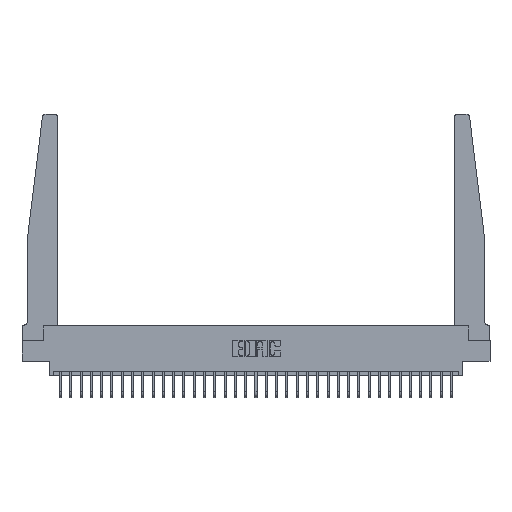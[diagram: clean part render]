
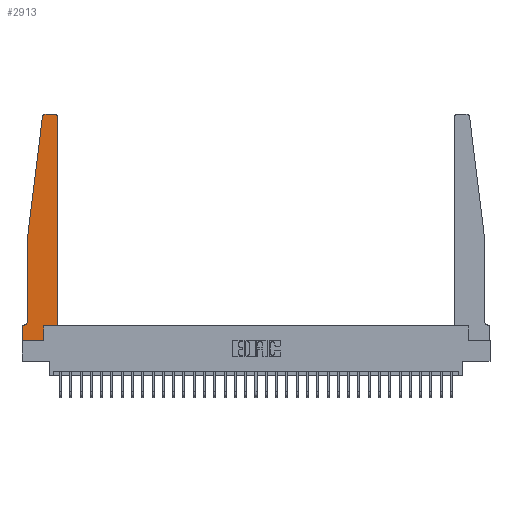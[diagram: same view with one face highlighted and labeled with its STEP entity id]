
A CAD part, top view. The second image highlights one B-rep face of the part: STEP entity #2913.
In plain terms, the highlighted planar face has unit normal (0, 0, 1).
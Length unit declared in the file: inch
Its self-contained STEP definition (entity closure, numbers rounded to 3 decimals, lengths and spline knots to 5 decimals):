
#86 = VERTEX_POINT ( 'NONE', #5348 ) ;
#124 = EDGE_CURVE ( 'NONE', #28373, #17568, #4726, .T. ) ;
#569 = CARTESIAN_POINT ( 'NONE',  ( 0.425, 0.18, 0.37 ) ) ;
#706 = VECTOR ( 'NONE', #23065, 39.37008 ) ;
#1404 = DIRECTION ( 'NONE',  ( -0.122, -0.992, 0. ) ) ;
#1860 = VERTEX_POINT ( 'NONE', #11119 ) ;
#1954 = LINE ( 'NONE', #28552, #3933 ) ;
#2847 = CARTESIAN_POINT ( 'NONE',  ( 0.015, 0.1875, 0.37 ) ) ;
#2901 = EDGE_CURVE ( 'NONE', #11012, #7720, #5055, .T. ) ;
#2913 = ADVANCED_FACE ( 'NONE', ( #12912 ), #19664, .T. ) ;
#3160 = CARTESIAN_POINT ( 'NONE',  ( 0., 0., 0.37 ) ) ;
#3933 = VECTOR ( 'NONE', #21158, 39.37008 ) ;
#4501 = CARTESIAN_POINT ( 'NONE',  ( 0.25, 2.75, 0.37 ) ) ;
#4514 = DIRECTION ( 'NONE',  ( 0., 0., 1. ) ) ;
#4726 = LINE ( 'NONE', #18181, #706 ) ;
#5055 = CIRCLE ( 'NONE', #15534, 0.03 ) ;
#5106 = EDGE_CURVE ( 'NONE', #86, #31598, #19056, .T. ) ;
#5206 = EDGE_CURVE ( 'NONE', #7720, #86, #7286, .T. ) ;
#5348 = CARTESIAN_POINT ( 'NONE',  ( 0.065, 1.25, 0.37 ) ) ;
#5720 = VECTOR ( 'NONE', #13809, 39.37008 ) ;
#5802 = ORIENTED_EDGE ( 'NONE', *, *, #2901, .T. ) ;
#5968 = LINE ( 'NONE', #26491, #18101 ) ;
#6328 = DIRECTION ( 'NONE',  ( 0., -1., 0. ) ) ;
#6398 = ORIENTED_EDGE ( 'NONE', *, *, #15980, .T. ) ;
#7286 = LINE ( 'NONE', #26779, #8465 ) ;
#7720 = VERTEX_POINT ( 'NONE', #19216 ) ;
#7993 = EDGE_CURVE ( 'NONE', #17568, #1860, #5968, .T. ) ;
#8465 = VECTOR ( 'NONE', #1404, 39.37008 ) ;
#8578 = VERTEX_POINT ( 'NONE', #11806 ) ;
#9713 = CARTESIAN_POINT ( 'NONE',  ( 0.27653, 2.72, 0.37 ) ) ;
#10337 = VECTOR ( 'NONE', #14319, 39.37008 ) ;
#11012 = VERTEX_POINT ( 'NONE', #11252 ) ;
#11119 = CARTESIAN_POINT ( 'NONE',  ( 0.2605, 0.18, 0.37 ) ) ;
#11252 = CARTESIAN_POINT ( 'NONE',  ( 0.27653, 2.75, 0.37 ) ) ;
#11569 = VECTOR ( 'NONE', #6328, 39.37008 ) ;
#11806 = CARTESIAN_POINT ( 'NONE',  ( 0., 0.1875, 0.37 ) ) ;
#12912 = FACE_OUTER_BOUND ( 'NONE', #17533, .T. ) ;
#13476 = CARTESIAN_POINT ( 'NONE',  ( 0.395, 2.72, 0.37 ) ) ;
#13585 = CARTESIAN_POINT ( 'NONE',  ( 0.065, 0.1875, 0.37 ) ) ;
#13733 = VECTOR ( 'NONE', #22242, 39.37008 ) ;
#13809 = DIRECTION ( 'NONE',  ( -1., 0., 0. ) ) ;
#14262 = ORIENTED_EDGE ( 'NONE', *, *, #5106, .T. ) ;
#14319 = DIRECTION ( 'NONE',  ( -1., 0., 0. ) ) ;
#14444 = EDGE_CURVE ( 'NONE', #18165, #8578, #19824, .T. ) ;
#15166 = AXIS2_PLACEMENT_3D ( 'NONE', #13476, #28771, #18740 ) ;
#15534 = AXIS2_PLACEMENT_3D ( 'NONE', #9713, #21860, #27191 ) ;
#15980 = EDGE_CURVE ( 'NONE', #24238, #24051, #32244, .T. ) ;
#15991 = EDGE_CURVE ( 'NONE', #1860, #20395, #1954, .T. ) ;
#16553 = LINE ( 'NONE', #32481, #21638 ) ;
#17031 = LINE ( 'NONE', #4501, #10337 ) ;
#17262 = DIRECTION ( 'NONE',  ( 0., -1., 0. ) ) ;
#17533 = EDGE_LOOP ( 'NONE', ( #22531, #5802, #19199, #14262, #23984, #23896, #27228, #31394, #29943, #26970, #26092, #6398 ) ) ;
#17568 = VERTEX_POINT ( 'NONE', #26055 ) ;
#17619 = EDGE_CURVE ( 'NONE', #20395, #24238, #21198, .T. ) ;
#18101 = VECTOR ( 'NONE', #26188, 39.37008 ) ;
#18165 = VERTEX_POINT ( 'NONE', #2847 ) ;
#18181 = CARTESIAN_POINT ( 'NONE',  ( 0., 0., 0.37 ) ) ;
#18399 = CARTESIAN_POINT ( 'NONE',  ( 0.065, 1.25, 0.37 ) ) ;
#18740 = DIRECTION ( 'NONE',  ( 1., 0., 0. ) ) ;
#19056 = LINE ( 'NONE', #18399, #11569 ) ;
#19199 = ORIENTED_EDGE ( 'NONE', *, *, #5206, .T. ) ;
#19216 = CARTESIAN_POINT ( 'NONE',  ( 0.24675, 2.72367, 0.37 ) ) ;
#19609 = DIRECTION ( 'NONE',  ( -1., 0., 0. ) ) ;
#19664 = PLANE ( 'NONE',  #32351 ) ;
#19824 = LINE ( 'NONE', #13585, #5720 ) ;
#20395 = VERTEX_POINT ( 'NONE', #569 ) ;
#21158 = DIRECTION ( 'NONE',  ( 1., 0., 0. ) ) ;
#21198 = LINE ( 'NONE', #28609, #13733 ) ;
#21379 = AXIS2_PLACEMENT_3D ( 'NONE', #27125, #32226, #19609 ) ;
#21638 = VECTOR ( 'NONE', #17262, 39.37008 ) ;
#21860 = DIRECTION ( 'NONE',  ( 0., 0., 1. ) ) ;
#22242 = DIRECTION ( 'NONE',  ( 0., 1., 0. ) ) ;
#22456 = CARTESIAN_POINT ( 'NONE',  ( 0.425, 2.72, 0.37 ) ) ;
#22531 = ORIENTED_EDGE ( 'NONE', *, *, #31388, .T. ) ;
#22738 = CARTESIAN_POINT ( 'NONE',  ( 0.065, 0.2375, 0.37 ) ) ;
#22849 = CIRCLE ( 'NONE', #21379, 0.05 ) ;
#23065 = DIRECTION ( 'NONE',  ( 1., 0., 0. ) ) ;
#23896 = ORIENTED_EDGE ( 'NONE', *, *, #14444, .T. ) ;
#23984 = ORIENTED_EDGE ( 'NONE', *, *, #30453, .T. ) ;
#24051 = VERTEX_POINT ( 'NONE', #24077 ) ;
#24077 = CARTESIAN_POINT ( 'NONE',  ( 0.395, 2.75, 0.37 ) ) ;
#24238 = VERTEX_POINT ( 'NONE', #22456 ) ;
#24707 = DIRECTION ( 'NONE',  ( 1., 0., 0. ) ) ;
#26055 = CARTESIAN_POINT ( 'NONE',  ( 0.2605, 0., 0.37 ) ) ;
#26092 = ORIENTED_EDGE ( 'NONE', *, *, #17619, .T. ) ;
#26188 = DIRECTION ( 'NONE',  ( 0., 1., 0. ) ) ;
#26491 = CARTESIAN_POINT ( 'NONE',  ( 0.2605, 0.18, 0.37 ) ) ;
#26779 = CARTESIAN_POINT ( 'NONE',  ( 0.065, 1.25, 0.37 ) ) ;
#26970 = ORIENTED_EDGE ( 'NONE', *, *, #15991, .T. ) ;
#27125 = CARTESIAN_POINT ( 'NONE',  ( 0.015, 0.2375, 0.37 ) ) ;
#27191 = DIRECTION ( 'NONE',  ( 1., 0., 0. ) ) ;
#27228 = ORIENTED_EDGE ( 'NONE', *, *, #32197, .T. ) ;
#28373 = VERTEX_POINT ( 'NONE', #3160 ) ;
#28552 = CARTESIAN_POINT ( 'NONE',  ( 0.425, 0.18, 0.37 ) ) ;
#28609 = CARTESIAN_POINT ( 'NONE',  ( 0.425, 0.18, 0.37 ) ) ;
#28771 = DIRECTION ( 'NONE',  ( 0., 0., 1. ) ) ;
#29731 = CARTESIAN_POINT ( 'NONE',  ( 0., 0.1875, 0.37 ) ) ;
#29943 = ORIENTED_EDGE ( 'NONE', *, *, #7993, .T. ) ;
#30453 = EDGE_CURVE ( 'NONE', #31598, #18165, #22849, .T. ) ;
#31388 = EDGE_CURVE ( 'NONE', #24051, #11012, #17031, .T. ) ;
#31394 = ORIENTED_EDGE ( 'NONE', *, *, #124, .T. ) ;
#31598 = VERTEX_POINT ( 'NONE', #22738 ) ;
#32197 = EDGE_CURVE ( 'NONE', #8578, #28373, #16553, .T. ) ;
#32226 = DIRECTION ( 'NONE',  ( 0., 0., -1. ) ) ;
#32244 = CIRCLE ( 'NONE', #15166, 0.03 ) ;
#32351 = AXIS2_PLACEMENT_3D ( 'NONE', #29731, #4514, #24707 ) ;
#32481 = CARTESIAN_POINT ( 'NONE',  ( 0., 0., 0.37 ) ) ;
